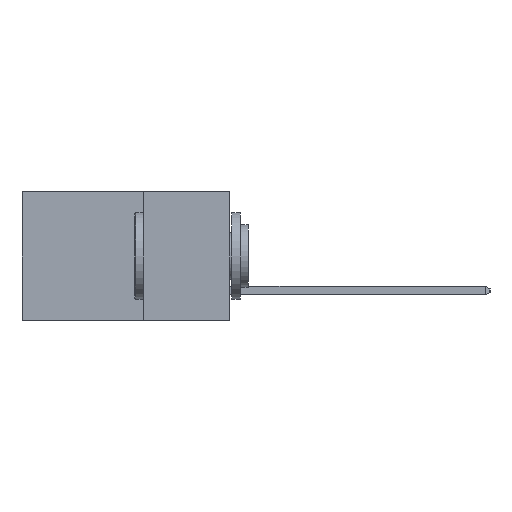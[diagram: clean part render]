
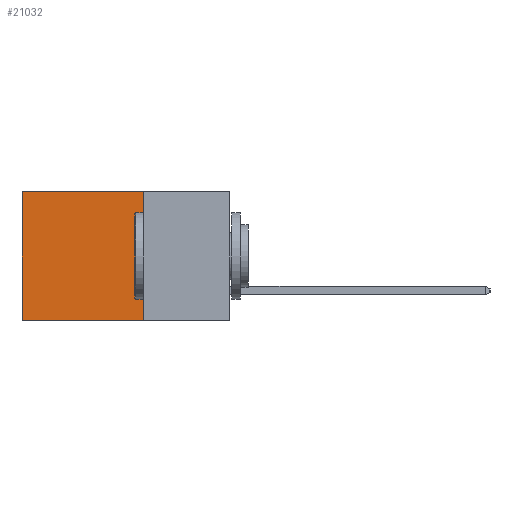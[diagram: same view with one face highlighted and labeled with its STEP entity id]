
A CAD part, left-side view. The second image highlights one B-rep face of the part: STEP entity #21032.
In plain terms, the highlighted planar face has unit normal (-1, 0, 0).
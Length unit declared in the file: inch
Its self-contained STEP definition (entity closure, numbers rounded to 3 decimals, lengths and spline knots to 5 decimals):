
#207 = VECTOR ( 'NONE', #8286, 39.37008 ) ;
#2377 = DIRECTION ( 'NONE',  ( 0., 1., 0. ) ) ;
#3716 = CARTESIAN_POINT ( 'NONE',  ( 0.2615, 0.25, -0.37 ) ) ;
#5050 = CARTESIAN_POINT ( 'NONE',  ( 0.2615, 0.25, -0.37 ) ) ;
#5052 = DIRECTION ( 'NONE',  ( 0., 0., -1. ) ) ;
#5529 = CARTESIAN_POINT ( 'NONE',  ( 0.2615, 0.6, 0. ) ) ;
#5892 = ORIENTED_EDGE ( 'NONE', *, *, #7281, .T. ) ;
#7200 = VERTEX_POINT ( 'NONE', #22178 ) ;
#7281 = EDGE_CURVE ( 'NONE', #7200, #24123, #15223, .T. ) ;
#7614 = EDGE_CURVE ( 'NONE', #19858, #18611, #8571, .T. ) ;
#8282 = CARTESIAN_POINT ( 'NONE',  ( 0.2615, 0.6, -0.37 ) ) ;
#8286 = DIRECTION ( 'NONE',  ( 0., 0., -1. ) ) ;
#8411 = ORIENTED_EDGE ( 'NONE', *, *, #7614, .F. ) ;
#8571 = LINE ( 'NONE', #3716, #11912 ) ;
#8803 = AXIS2_PLACEMENT_3D ( 'NONE', #8977, #22132, #10915 ) ;
#8977 = CARTESIAN_POINT ( 'NONE',  ( 0.2615, 0.25, -0.37 ) ) ;
#9141 = EDGE_LOOP ( 'NONE', ( #21909, #8411, #10864, #5892 ) ) ;
#10042 = LINE ( 'NONE', #8282, #207 ) ;
#10102 = VECTOR ( 'NONE', #16885, 39.37008 ) ;
#10864 = ORIENTED_EDGE ( 'NONE', *, *, #11998, .F. ) ;
#10915 = DIRECTION ( 'NONE',  ( 0., 0., -1. ) ) ;
#11912 = VECTOR ( 'NONE', #2377, 39.37008 ) ;
#11998 = EDGE_CURVE ( 'NONE', #7200, #19858, #17632, .T. ) ;
#12591 = VECTOR ( 'NONE', #5052, 39.37008 ) ;
#13642 = FACE_OUTER_BOUND ( 'NONE', #9141, .T. ) ;
#14675 = EDGE_CURVE ( 'NONE', #24123, #18611, #10042, .T. ) ;
#15223 = LINE ( 'NONE', #17822, #10102 ) ;
#16619 = CARTESIAN_POINT ( 'NONE',  ( 0.2615, 0.25, -0.37 ) ) ;
#16885 = DIRECTION ( 'NONE',  ( 0., 1., 0. ) ) ;
#17632 = LINE ( 'NONE', #5050, #12591 ) ;
#17822 = CARTESIAN_POINT ( 'NONE',  ( 0.2615, 0.25, 0. ) ) ;
#18437 = PLANE ( 'NONE',  #8803 ) ;
#18611 = VERTEX_POINT ( 'NONE', #19197 ) ;
#19197 = CARTESIAN_POINT ( 'NONE',  ( 0.2615, 0.6, -0.37 ) ) ;
#19858 = VERTEX_POINT ( 'NONE', #16619 ) ;
#21032 = ADVANCED_FACE ( 'NONE', ( #13642 ), #18437, .F. ) ;
#21909 = ORIENTED_EDGE ( 'NONE', *, *, #14675, .T. ) ;
#22132 = DIRECTION ( 'NONE',  ( 1., 0., 0. ) ) ;
#22178 = CARTESIAN_POINT ( 'NONE',  ( 0.2615, 0.25, 0. ) ) ;
#24123 = VERTEX_POINT ( 'NONE', #5529 ) ;
